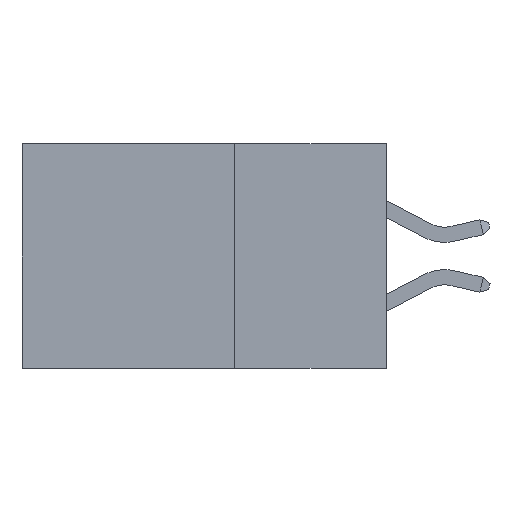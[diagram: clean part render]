
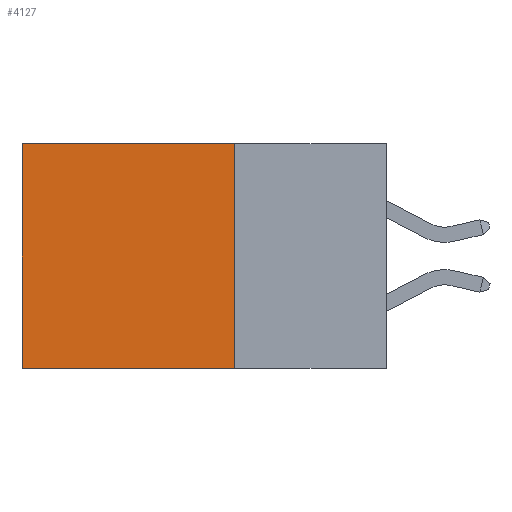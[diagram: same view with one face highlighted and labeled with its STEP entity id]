
A CAD part, left-side view. The second image highlights one B-rep face of the part: STEP entity #4127.
In plain terms, the highlighted planar face has unit normal (-1, 0, 0).
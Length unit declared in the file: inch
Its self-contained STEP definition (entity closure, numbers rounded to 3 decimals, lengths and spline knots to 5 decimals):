
#165 = ORIENTED_EDGE ( 'NONE', *, *, #3481, .F. ) ;
#207 = VERTEX_POINT ( 'NONE', #4244 ) ;
#1341 = CARTESIAN_POINT ( 'NONE',  ( 0.2615, 0.25, 0. ) ) ;
#1454 = CARTESIAN_POINT ( 'NONE',  ( 0.2615, 0.25, 0. ) ) ;
#1871 = EDGE_LOOP ( 'NONE', ( #10088, #5615, #165, #5980 ) ) ;
#2067 = CARTESIAN_POINT ( 'NONE',  ( 0.2615, 0.25, -0.37 ) ) ;
#2145 = VECTOR ( 'NONE', #3026, 39.37008 ) ;
#2352 = EDGE_CURVE ( 'NONE', #9782, #10083, #10159, .T. ) ;
#2401 = EDGE_CURVE ( 'NONE', #207, #10083, #9016, .T. ) ;
#2797 = CARTESIAN_POINT ( 'NONE',  ( 0.2615, 0.25, -0.37 ) ) ;
#3026 = DIRECTION ( 'NONE',  ( 0., 0., -1. ) ) ;
#3481 = EDGE_CURVE ( 'NONE', #7713, #207, #8389, .T. ) ;
#3904 = LINE ( 'NONE', #1454, #7671 ) ;
#4127 = ADVANCED_FACE ( 'NONE', ( #4985 ), #10357, .F. ) ;
#4244 = CARTESIAN_POINT ( 'NONE',  ( 0.2615, 0.25, -0.37 ) ) ;
#4258 = VECTOR ( 'NONE', #8652, 39.37008 ) ;
#4481 = DIRECTION ( 'NONE',  ( 1., 0., 0. ) ) ;
#4985 = FACE_OUTER_BOUND ( 'NONE', #1871, .T. ) ;
#5615 = ORIENTED_EDGE ( 'NONE', *, *, #2401, .F. ) ;
#5717 = EDGE_CURVE ( 'NONE', #7713, #9782, #3904, .T. ) ;
#5980 = ORIENTED_EDGE ( 'NONE', *, *, #5717, .T. ) ;
#5981 = CARTESIAN_POINT ( 'NONE',  ( 0.2615, 0.6, -0.37 ) ) ;
#6227 = AXIS2_PLACEMENT_3D ( 'NONE', #2797, #4481, #9663 ) ;
#7671 = VECTOR ( 'NONE', #7883, 39.37008 ) ;
#7713 = VERTEX_POINT ( 'NONE', #1341 ) ;
#7883 = DIRECTION ( 'NONE',  ( 0., 1., 0. ) ) ;
#8000 = DIRECTION ( 'NONE',  ( 0., 1., 0. ) ) ;
#8041 = CARTESIAN_POINT ( 'NONE',  ( 0.2615, 0.25, -0.37 ) ) ;
#8389 = LINE ( 'NONE', #2067, #2145 ) ;
#8502 = CARTESIAN_POINT ( 'NONE',  ( 0.2615, 0.6, 0. ) ) ;
#8652 = DIRECTION ( 'NONE',  ( 0., 0., -1. ) ) ;
#8663 = CARTESIAN_POINT ( 'NONE',  ( 0.2615, 0.6, -0.37 ) ) ;
#8774 = VECTOR ( 'NONE', #8000, 39.37008 ) ;
#9016 = LINE ( 'NONE', #8041, #8774 ) ;
#9663 = DIRECTION ( 'NONE',  ( 0., 0., -1. ) ) ;
#9782 = VERTEX_POINT ( 'NONE', #8502 ) ;
#10083 = VERTEX_POINT ( 'NONE', #5981 ) ;
#10088 = ORIENTED_EDGE ( 'NONE', *, *, #2352, .T. ) ;
#10159 = LINE ( 'NONE', #8663, #4258 ) ;
#10357 = PLANE ( 'NONE',  #6227 ) ;
